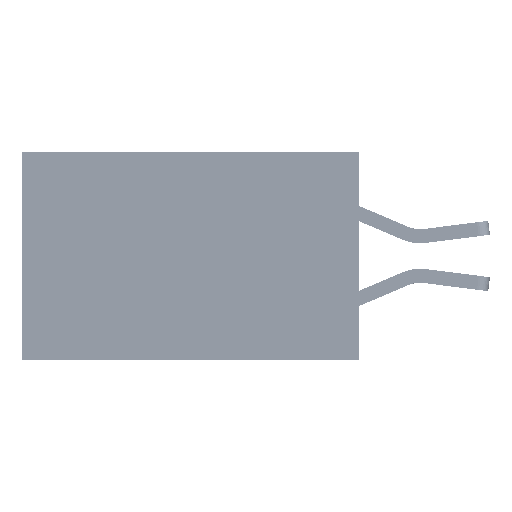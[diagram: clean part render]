
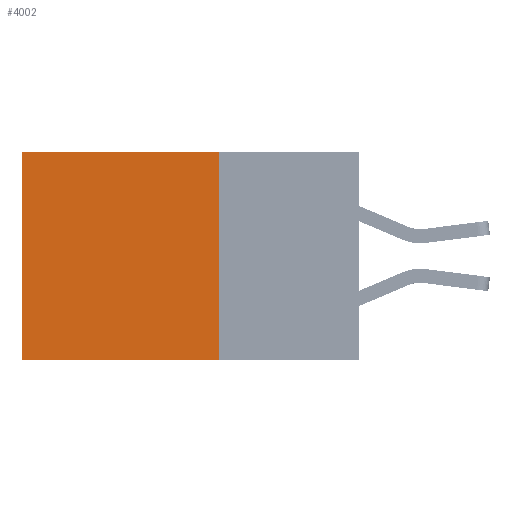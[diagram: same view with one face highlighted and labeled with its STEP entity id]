
A CAD part, left-side view. The second image highlights one B-rep face of the part: STEP entity #4002.
In plain terms, the highlighted planar face has unit normal (-1, 0, 0).
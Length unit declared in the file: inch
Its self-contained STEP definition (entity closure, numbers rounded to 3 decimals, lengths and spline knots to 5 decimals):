
#1739 = ORIENTED_EDGE ( 'NONE', *, *, #16846, .F. ) ;
#2167 = CARTESIAN_POINT ( 'NONE',  ( 0.2875, 0.25, 0. ) ) ;
#2471 = VERTEX_POINT ( 'NONE', #36666 ) ;
#3486 = CARTESIAN_POINT ( 'NONE',  ( 0.2875, 0.25, 0. ) ) ;
#4002 = ADVANCED_FACE ( 'NONE', ( #25687 ), #46782, .F. ) ;
#4800 = CARTESIAN_POINT ( 'NONE',  ( 0.2875, 0.25, 0. ) ) ;
#5685 = VERTEX_POINT ( 'NONE', #41514 ) ;
#6125 = DIRECTION ( 'NONE',  ( 1., 0., 0. ) ) ;
#7388 = VECTOR ( 'NONE', #41755, 39.37008 ) ;
#8047 = ORIENTED_EDGE ( 'NONE', *, *, #45248, .F. ) ;
#8727 = DIRECTION ( 'NONE',  ( 0., 1., 0. ) ) ;
#9116 = LINE ( 'NONE', #3486, #46085 ) ;
#9801 = LINE ( 'NONE', #19623, #7388 ) ;
#14166 = EDGE_LOOP ( 'NONE', ( #23907, #1739, #8047, #45121 ) ) ;
#14363 = LINE ( 'NONE', #4800, #32890 ) ;
#16846 = EDGE_CURVE ( 'NONE', #5685, #17793, #28938, .T. ) ;
#17793 = VERTEX_POINT ( 'NONE', #30808 ) ;
#19623 = CARTESIAN_POINT ( 'NONE',  ( 0.2875, 0.6, 0. ) ) ;
#21863 = CARTESIAN_POINT ( 'NONE',  ( 0.2875, 0.25, -0.37 ) ) ;
#23907 = ORIENTED_EDGE ( 'NONE', *, *, #29187, .T. ) ;
#25687 = FACE_OUTER_BOUND ( 'NONE', #14166, .T. ) ;
#26043 = CARTESIAN_POINT ( 'NONE',  ( 0.2875, 0.25, 0. ) ) ;
#27782 = VECTOR ( 'NONE', #36466, 39.37008 ) ;
#28938 = LINE ( 'NONE', #21863, #27782 ) ;
#29187 = EDGE_CURVE ( 'NONE', #2471, #17793, #9801, .T. ) ;
#30808 = CARTESIAN_POINT ( 'NONE',  ( 0.2875, 0.6, -0.37 ) ) ;
#31261 = AXIS2_PLACEMENT_3D ( 'NONE', #2167, #6125, #32265 ) ;
#32265 = DIRECTION ( 'NONE',  ( 0., 0., -1. ) ) ;
#32890 = VECTOR ( 'NONE', #8727, 39.37008 ) ;
#33482 = DIRECTION ( 'NONE',  ( 0., 0., -1. ) ) ;
#36466 = DIRECTION ( 'NONE',  ( 0., 1., 0. ) ) ;
#36666 = CARTESIAN_POINT ( 'NONE',  ( 0.2875, 0.6, 0. ) ) ;
#37048 = EDGE_CURVE ( 'NONE', #44608, #2471, #14363, .T. ) ;
#41514 = CARTESIAN_POINT ( 'NONE',  ( 0.2875, 0.25, -0.37 ) ) ;
#41755 = DIRECTION ( 'NONE',  ( 0., 0., -1. ) ) ;
#44608 = VERTEX_POINT ( 'NONE', #26043 ) ;
#45121 = ORIENTED_EDGE ( 'NONE', *, *, #37048, .T. ) ;
#45248 = EDGE_CURVE ( 'NONE', #44608, #5685, #9116, .T. ) ;
#46085 = VECTOR ( 'NONE', #33482, 39.37008 ) ;
#46782 = PLANE ( 'NONE',  #31261 ) ;
